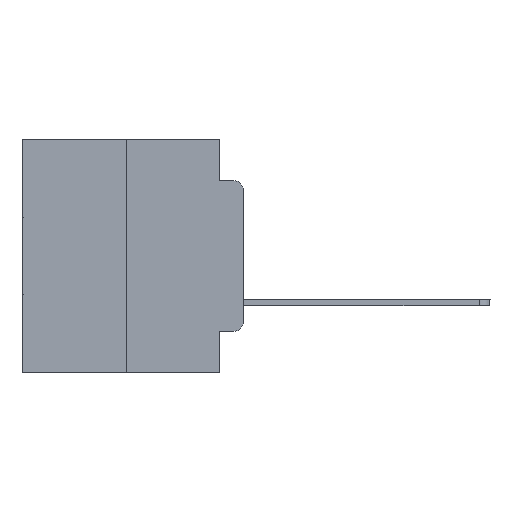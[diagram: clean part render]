
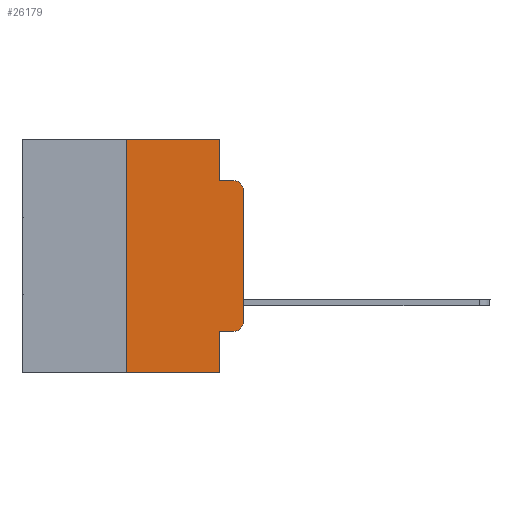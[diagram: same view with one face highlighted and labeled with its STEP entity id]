
A CAD part, left-side view. The second image highlights one B-rep face of the part: STEP entity #26179.
In plain terms, the highlighted planar face has unit normal (-1, 0, 0).
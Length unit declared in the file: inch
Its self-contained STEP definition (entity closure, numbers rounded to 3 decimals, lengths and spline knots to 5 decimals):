
#432 = ORIENTED_EDGE ( 'NONE', *, *, #24447, .F. ) ;
#721 = CARTESIAN_POINT ( 'NONE',  ( 0., 0., -0.1085 ) ) ;
#1266 = DIRECTION ( 'NONE',  ( 0., -1., 0. ) ) ;
#1406 = LINE ( 'NONE', #12455, #18266 ) ;
#1927 = CARTESIAN_POINT ( 'NONE',  ( 0., 0., 0. ) ) ;
#2723 = CARTESIAN_POINT ( 'NONE',  ( 0., 0.02, -0.3915 ) ) ;
#2739 = DIRECTION ( 'NONE',  ( 0., -1., 0. ) ) ;
#3212 = VERTEX_POINT ( 'NONE', #18770 ) ;
#3275 = VECTOR ( 'NONE', #9411, 39.37008 ) ;
#3374 = AXIS2_PLACEMENT_3D ( 'NONE', #2723, #11415, #11713 ) ;
#3410 = CARTESIAN_POINT ( 'NONE',  ( 0., 0.02, -0.1085 ) ) ;
#3556 = VERTEX_POINT ( 'NONE', #11104 ) ;
#4382 = CARTESIAN_POINT ( 'NONE',  ( 0., 0.473, 0. ) ) ;
#4466 = VECTOR ( 'NONE', #6070, 39.37008 ) ;
#4618 = VECTOR ( 'NONE', #2739, 39.37008 ) ;
#4783 = CARTESIAN_POINT ( 'NONE',  ( 0., 0.02, -0.0885 ) ) ;
#4989 = LINE ( 'NONE', #27636, #3275 ) ;
#5383 = EDGE_CURVE ( 'NONE', #15999, #15087, #22102, .T. ) ;
#5923 = CARTESIAN_POINT ( 'NONE',  ( 0., 0.25, 0. ) ) ;
#6070 = DIRECTION ( 'NONE',  ( 0., 0., 1. ) ) ;
#6487 = ORIENTED_EDGE ( 'NONE', *, *, #22042, .F. ) ;
#6595 = EDGE_LOOP ( 'NONE', ( #25870, #26302, #6487, #8913, #432, #13640, #27209, #17660, #16230, #11238 ) ) ;
#6778 = VERTEX_POINT ( 'NONE', #8573 ) ;
#8573 = CARTESIAN_POINT ( 'NONE',  ( 0., 0.02, -0.4115 ) ) ;
#8913 = ORIENTED_EDGE ( 'NONE', *, *, #9305, .F. ) ;
#9305 = EDGE_CURVE ( 'NONE', #26037, #21030, #26525, .T. ) ;
#9411 = DIRECTION ( 'NONE',  ( 0., -1., 0. ) ) ;
#9543 = PLANE ( 'NONE',  #25914 ) ;
#9646 = EDGE_CURVE ( 'NONE', #13098, #3212, #27833, .T. ) ;
#11104 = CARTESIAN_POINT ( 'NONE',  ( 0., 0.051, -0.4115 ) ) ;
#11238 = ORIENTED_EDGE ( 'NONE', *, *, #27788, .T. ) ;
#11415 = DIRECTION ( 'NONE',  ( -1., 0., 0. ) ) ;
#11713 = DIRECTION ( 'NONE',  ( 0., 0., -1. ) ) ;
#12455 = CARTESIAN_POINT ( 'NONE',  ( 0., 0.473, -0.5 ) ) ;
#12820 = LINE ( 'NONE', #26056, #20220 ) ;
#12972 = DIRECTION ( 'NONE',  ( 0., 0., -1. ) ) ;
#13098 = VERTEX_POINT ( 'NONE', #25490 ) ;
#13233 = CIRCLE ( 'NONE', #14166, 0.02 ) ;
#13640 = ORIENTED_EDGE ( 'NONE', *, *, #9646, .F. ) ;
#14075 = VECTOR ( 'NONE', #26813, 39.37008 ) ;
#14166 = AXIS2_PLACEMENT_3D ( 'NONE', #3410, #26208, #12972 ) ;
#15026 = VECTOR ( 'NONE', #21363, 39.37008 ) ;
#15087 = VERTEX_POINT ( 'NONE', #721 ) ;
#15185 = CARTESIAN_POINT ( 'NONE',  ( 0., 0.051, -0.5 ) ) ;
#15654 = CARTESIAN_POINT ( 'NONE',  ( 0., 0.051, -0.0885 ) ) ;
#15999 = VERTEX_POINT ( 'NONE', #16251 ) ;
#16230 = ORIENTED_EDGE ( 'NONE', *, *, #26328, .T. ) ;
#16251 = CARTESIAN_POINT ( 'NONE',  ( 0., 0., -0.3915 ) ) ;
#16680 = EDGE_CURVE ( 'NONE', #3556, #18013, #12820, .T. ) ;
#17091 = DIRECTION ( 'NONE',  ( 0., 0., -1. ) ) ;
#17634 = CARTESIAN_POINT ( 'NONE',  ( 0., 0.051, 0. ) ) ;
#17660 = ORIENTED_EDGE ( 'NONE', *, *, #16680, .F. ) ;
#17910 = FACE_OUTER_BOUND ( 'NONE', #6595, .T. ) ;
#18013 = VERTEX_POINT ( 'NONE', #15185 ) ;
#18266 = VECTOR ( 'NONE', #19360, 39.37008 ) ;
#18770 = CARTESIAN_POINT ( 'NONE',  ( 0., 0.25, 0. ) ) ;
#19360 = DIRECTION ( 'NONE',  ( 0., -1., 0. ) ) ;
#19630 = CARTESIAN_POINT ( 'NONE',  ( 0., 0.051, 0. ) ) ;
#20220 = VECTOR ( 'NONE', #17091, 39.37008 ) ;
#20417 = DIRECTION ( 'NONE',  ( 1., 0., 0. ) ) ;
#21030 = VERTEX_POINT ( 'NONE', #15654 ) ;
#21363 = DIRECTION ( 'NONE',  ( 0., 0., 1. ) ) ;
#22042 = EDGE_CURVE ( 'NONE', #21030, #25361, #27745, .T. ) ;
#22102 = LINE ( 'NONE', #1927, #4466 ) ;
#22926 = DIRECTION ( 'NONE',  ( 0., 0., -1. ) ) ;
#23137 = VECTOR ( 'NONE', #1266, 39.37008 ) ;
#23219 = CARTESIAN_POINT ( 'NONE',  ( 0., 0.051, -0.4115 ) ) ;
#23344 = CARTESIAN_POINT ( 'NONE',  ( 0., 0.051, -0.0885 ) ) ;
#23360 = LINE ( 'NONE', #23219, #23137 ) ;
#23523 = EDGE_CURVE ( 'NONE', #13098, #18013, #1406, .T. ) ;
#24447 = EDGE_CURVE ( 'NONE', #3212, #26037, #4989, .T. ) ;
#24988 = CIRCLE ( 'NONE', #3374, 0.02 ) ;
#25361 = VERTEX_POINT ( 'NONE', #4783 ) ;
#25490 = CARTESIAN_POINT ( 'NONE',  ( 0., 0.25, -0.5 ) ) ;
#25870 = ORIENTED_EDGE ( 'NONE', *, *, #5383, .T. ) ;
#25914 = AXIS2_PLACEMENT_3D ( 'NONE', #4382, #20417, #22926 ) ;
#26037 = VERTEX_POINT ( 'NONE', #17634 ) ;
#26056 = CARTESIAN_POINT ( 'NONE',  ( 0., 0.051, 0. ) ) ;
#26179 = ADVANCED_FACE ( 'NONE', ( #17910 ), #9543, .F. ) ;
#26208 = DIRECTION ( 'NONE',  ( -1., 0., 0. ) ) ;
#26302 = ORIENTED_EDGE ( 'NONE', *, *, #27329, .T. ) ;
#26328 = EDGE_CURVE ( 'NONE', #3556, #6778, #23360, .T. ) ;
#26525 = LINE ( 'NONE', #19630, #14075 ) ;
#26813 = DIRECTION ( 'NONE',  ( 0., 0., -1. ) ) ;
#27209 = ORIENTED_EDGE ( 'NONE', *, *, #23523, .T. ) ;
#27329 = EDGE_CURVE ( 'NONE', #15087, #25361, #13233, .T. ) ;
#27636 = CARTESIAN_POINT ( 'NONE',  ( 0., 0.473, 0. ) ) ;
#27745 = LINE ( 'NONE', #23344, #4618 ) ;
#27788 = EDGE_CURVE ( 'NONE', #6778, #15999, #24988, .T. ) ;
#27833 = LINE ( 'NONE', #5923, #15026 ) ;
